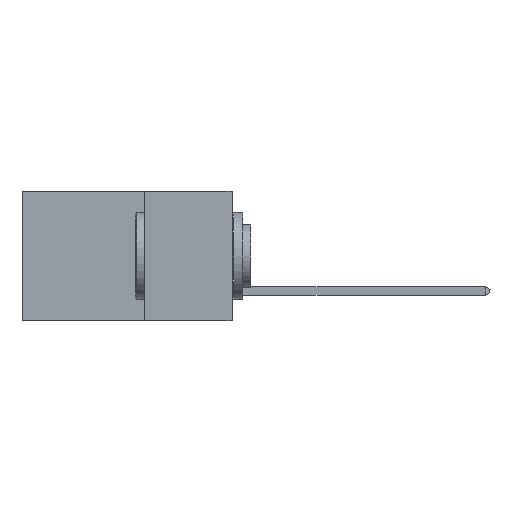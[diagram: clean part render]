
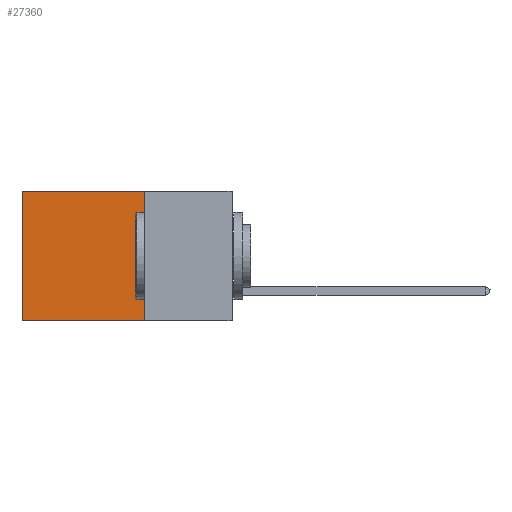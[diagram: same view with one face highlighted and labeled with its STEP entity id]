
A CAD part, left-side view. The second image highlights one B-rep face of the part: STEP entity #27360.
In plain terms, the highlighted planar face has unit normal (-1, 0, 0).
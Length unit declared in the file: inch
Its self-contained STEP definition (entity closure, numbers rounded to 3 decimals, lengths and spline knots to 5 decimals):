
#453 = ORIENTED_EDGE ( 'NONE', *, *, #30371, .T. ) ;
#2504 = VERTEX_POINT ( 'NONE', #24191 ) ;
#3083 = VECTOR ( 'NONE', #18238, 39.37008 ) ;
#8025 = VERTEX_POINT ( 'NONE', #31778 ) ;
#8043 = PLANE ( 'NONE',  #38638 ) ;
#8597 = ORIENTED_EDGE ( 'NONE', *, *, #30451, .T. ) ;
#11845 = CARTESIAN_POINT ( 'NONE',  ( 0.2875, 0.6, 0. ) ) ;
#14866 = VECTOR ( 'NONE', #32484, 39.37008 ) ;
#18238 = DIRECTION ( 'NONE',  ( 0., 0., -1. ) ) ;
#18831 = DIRECTION ( 'NONE',  ( 0., 1., 0. ) ) ;
#19891 = CARTESIAN_POINT ( 'NONE',  ( 0.2875, 0.25, 0. ) ) ;
#20737 = FACE_OUTER_BOUND ( 'NONE', #31801, .T. ) ;
#22787 = LINE ( 'NONE', #24714, #14866 ) ;
#24191 = CARTESIAN_POINT ( 'NONE',  ( 0.2875, 0.6, -0.37 ) ) ;
#24714 = CARTESIAN_POINT ( 'NONE',  ( 0.2875, 0.6, 0. ) ) ;
#27360 = ADVANCED_FACE ( 'NONE', ( #20737 ), #8043, .F. ) ;
#28926 = DIRECTION ( 'NONE',  ( 0., 1., 0. ) ) ;
#30371 = EDGE_CURVE ( 'NONE', #8025, #44765, #43366, .T. ) ;
#30451 = EDGE_CURVE ( 'NONE', #44765, #2504, #22787, .T. ) ;
#30667 = EDGE_CURVE ( 'NONE', #8025, #37884, #35368, .T. ) ;
#31778 = CARTESIAN_POINT ( 'NONE',  ( 0.2875, 0.25, 0. ) ) ;
#31801 = EDGE_LOOP ( 'NONE', ( #8597, #48818, #32314, #453 ) ) ;
#32314 = ORIENTED_EDGE ( 'NONE', *, *, #30667, .F. ) ;
#32484 = DIRECTION ( 'NONE',  ( 0., 0., -1. ) ) ;
#33079 = VECTOR ( 'NONE', #28926, 39.37008 ) ;
#34471 = VECTOR ( 'NONE', #18831, 39.37008 ) ;
#35368 = LINE ( 'NONE', #45169, #3083 ) ;
#36050 = CARTESIAN_POINT ( 'NONE',  ( 0.2875, 0.25, 0. ) ) ;
#37884 = VERTEX_POINT ( 'NONE', #49049 ) ;
#38638 = AXIS2_PLACEMENT_3D ( 'NONE', #19891, #42609, #47169 ) ;
#42609 = DIRECTION ( 'NONE',  ( 1., 0., 0. ) ) ;
#43366 = LINE ( 'NONE', #36050, #33079 ) ;
#44765 = VERTEX_POINT ( 'NONE', #11845 ) ;
#44793 = LINE ( 'NONE', #50137, #34471 ) ;
#45169 = CARTESIAN_POINT ( 'NONE',  ( 0.2875, 0.25, 0. ) ) ;
#45293 = EDGE_CURVE ( 'NONE', #37884, #2504, #44793, .T. ) ;
#47169 = DIRECTION ( 'NONE',  ( 0., 0., -1. ) ) ;
#48818 = ORIENTED_EDGE ( 'NONE', *, *, #45293, .F. ) ;
#49049 = CARTESIAN_POINT ( 'NONE',  ( 0.2875, 0.25, -0.37 ) ) ;
#50137 = CARTESIAN_POINT ( 'NONE',  ( 0.2875, 0.25, -0.37 ) ) ;
